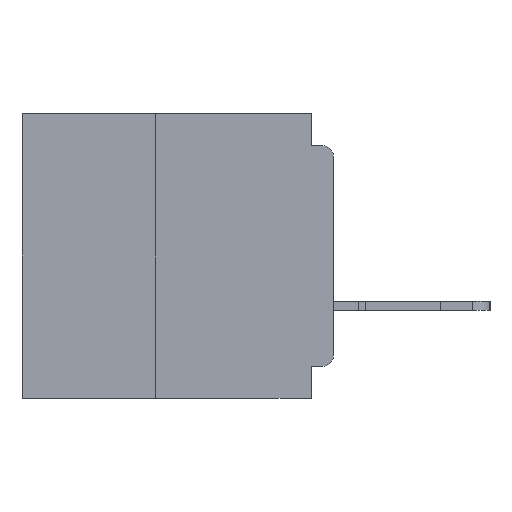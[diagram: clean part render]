
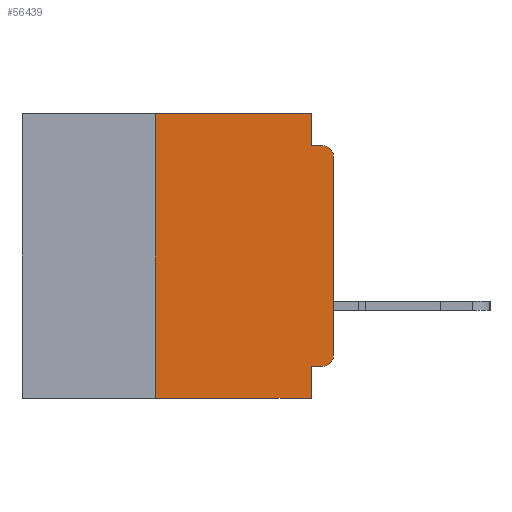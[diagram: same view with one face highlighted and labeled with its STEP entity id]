
A CAD part, left-side view. The second image highlights one B-rep face of the part: STEP entity #56439.
In plain terms, the highlighted planar face has unit normal (-1, 0, 0).
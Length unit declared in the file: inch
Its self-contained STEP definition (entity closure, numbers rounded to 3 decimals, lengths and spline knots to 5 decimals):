
#429 = CARTESIAN_POINT ( 'NONE',  ( 0., 0.015, -0.34 ) ) ;
#553 = EDGE_CURVE ( 'NONE', #53298, #14207, #32609, .T. ) ;
#2120 = PLANE ( 'NONE',  #48330 ) ;
#2488 = VERTEX_POINT ( 'NONE', #15504 ) ;
#4151 = FACE_OUTER_BOUND ( 'NONE', #9456, .T. ) ;
#4374 = ORIENTED_EDGE ( 'NONE', *, *, #48989, .F. ) ;
#4821 = CARTESIAN_POINT ( 'NONE',  ( 0., 0., -0.355 ) ) ;
#5250 = DIRECTION ( 'NONE',  ( 0., 0., -1. ) ) ;
#6593 = CARTESIAN_POINT ( 'NONE',  ( 0., 0., -0.34 ) ) ;
#6681 = VECTOR ( 'NONE', #27351, 39.37008 ) ;
#7150 = EDGE_CURVE ( 'NONE', #27262, #56945, #47640, .T. ) ;
#8183 = DIRECTION ( 'NONE',  ( -1., 0., 0. ) ) ;
#8783 = LINE ( 'NONE', #46534, #43451 ) ;
#9456 = EDGE_LOOP ( 'NONE', ( #33211, #60816, #21911, #58222, #13278, #57646, #57521, #50577, #4374, #11976 ) ) ;
#11715 = DIRECTION ( 'NONE',  ( 0., 0., -1. ) ) ;
#11976 = ORIENTED_EDGE ( 'NONE', *, *, #42810, .T. ) ;
#13278 = ORIENTED_EDGE ( 'NONE', *, *, #52804, .F. ) ;
#13912 = CARTESIAN_POINT ( 'NONE',  ( 0., 0.015, -0.045 ) ) ;
#14038 = VERTEX_POINT ( 'NONE', #56969 ) ;
#14207 = VERTEX_POINT ( 'NONE', #29874 ) ;
#15504 = CARTESIAN_POINT ( 'NONE',  ( 0., 0.031, -0.045 ) ) ;
#15814 = LINE ( 'NONE', #4821, #56228 ) ;
#18569 = VECTOR ( 'NONE', #18766, 39.37008 ) ;
#18766 = DIRECTION ( 'NONE',  ( 0., 0., 1. ) ) ;
#20874 = VECTOR ( 'NONE', #21956, 39.37008 ) ;
#21039 = DIRECTION ( 'NONE',  ( 0., -1., 0. ) ) ;
#21911 = ORIENTED_EDGE ( 'NONE', *, *, #32729, .F. ) ;
#21956 = DIRECTION ( 'NONE',  ( 0., -1., 0. ) ) ;
#22276 = CARTESIAN_POINT ( 'NONE',  ( 0., 0.25, -0.4 ) ) ;
#22679 = CIRCLE ( 'NONE', #32626, 0.015 ) ;
#27262 = VERTEX_POINT ( 'NONE', #22276 ) ;
#27351 = DIRECTION ( 'NONE',  ( 0., 0., 1. ) ) ;
#27953 = EDGE_CURVE ( 'NONE', #27262, #37650, #56746, .T. ) ;
#29874 = CARTESIAN_POINT ( 'NONE',  ( 0., 0., -0.06 ) ) ;
#30719 = CARTESIAN_POINT ( 'NONE',  ( 0., 0.031, -0.355 ) ) ;
#31317 = VECTOR ( 'NONE', #59017, 39.37008 ) ;
#31928 = CIRCLE ( 'NONE', #54908, 0.015 ) ;
#32609 = LINE ( 'NONE', #42254, #18569 ) ;
#32626 = AXIS2_PLACEMENT_3D ( 'NONE', #36455, #8183, #41176 ) ;
#32729 = EDGE_CURVE ( 'NONE', #2488, #40992, #33413, .T. ) ;
#33211 = ORIENTED_EDGE ( 'NONE', *, *, #553, .T. ) ;
#33413 = LINE ( 'NONE', #40703, #20874 ) ;
#33544 = DIRECTION ( 'NONE',  ( -1., 0., 0. ) ) ;
#35207 = CARTESIAN_POINT ( 'NONE',  ( 0., 0.437, 0. ) ) ;
#35329 = DIRECTION ( 'NONE',  ( 0., -1., 0. ) ) ;
#36455 = CARTESIAN_POINT ( 'NONE',  ( 0., 0.015, -0.06 ) ) ;
#36514 = VERTEX_POINT ( 'NONE', #30719 ) ;
#36623 = EDGE_CURVE ( 'NONE', #14207, #40992, #22679, .T. ) ;
#37320 = DIRECTION ( 'NONE',  ( 0., 0., -1. ) ) ;
#37650 = VERTEX_POINT ( 'NONE', #46918 ) ;
#37883 = DIRECTION ( 'NONE',  ( 0., 1., 0. ) ) ;
#39793 = CARTESIAN_POINT ( 'NONE',  ( 0., 0.437, -0.4 ) ) ;
#39947 = DIRECTION ( 'NONE',  ( 1., 0., 0. ) ) ;
#40005 = CARTESIAN_POINT ( 'NONE',  ( 0., 0.031, -0.4 ) ) ;
#40703 = CARTESIAN_POINT ( 'NONE',  ( 0., 0., -0.045 ) ) ;
#40992 = VERTEX_POINT ( 'NONE', #13912 ) ;
#41176 = DIRECTION ( 'NONE',  ( 0., 0., -1. ) ) ;
#42254 = CARTESIAN_POINT ( 'NONE',  ( 0., 0., 0. ) ) ;
#42810 = EDGE_CURVE ( 'NONE', #55442, #53298, #31928, .T. ) ;
#43451 = VECTOR ( 'NONE', #37320, 39.37008 ) ;
#43808 = LINE ( 'NONE', #40005, #31317 ) ;
#44564 = CARTESIAN_POINT ( 'NONE',  ( 0., 0.437, 0. ) ) ;
#46022 = CARTESIAN_POINT ( 'NONE',  ( 0., 0.25, -0.4 ) ) ;
#46534 = CARTESIAN_POINT ( 'NONE',  ( 0., 0.031, 0. ) ) ;
#46918 = CARTESIAN_POINT ( 'NONE',  ( 0., 0.25, 0. ) ) ;
#47640 = LINE ( 'NONE', #39793, #55677 ) ;
#48330 = AXIS2_PLACEMENT_3D ( 'NONE', #35207, #39947, #11715 ) ;
#48989 = EDGE_CURVE ( 'NONE', #55442, #36514, #15814, .T. ) ;
#50292 = CARTESIAN_POINT ( 'NONE',  ( 0., 0.015, -0.355 ) ) ;
#50577 = ORIENTED_EDGE ( 'NONE', *, *, #54080, .F. ) ;
#52804 = EDGE_CURVE ( 'NONE', #37650, #14038, #60818, .T. ) ;
#53298 = VERTEX_POINT ( 'NONE', #6593 ) ;
#54080 = EDGE_CURVE ( 'NONE', #36514, #56945, #43808, .T. ) ;
#54908 = AXIS2_PLACEMENT_3D ( 'NONE', #429, #33544, #5250 ) ;
#55442 = VERTEX_POINT ( 'NONE', #50292 ) ;
#55677 = VECTOR ( 'NONE', #21039, 39.37008 ) ;
#55811 = CARTESIAN_POINT ( 'NONE',  ( 0., 0.031, -0.4 ) ) ;
#56228 = VECTOR ( 'NONE', #37883, 39.37008 ) ;
#56439 = ADVANCED_FACE ( 'NONE', ( #4151 ), #2120, .F. ) ;
#56746 = LINE ( 'NONE', #46022, #6681 ) ;
#56945 = VERTEX_POINT ( 'NONE', #55811 ) ;
#56969 = CARTESIAN_POINT ( 'NONE',  ( 0., 0.031, 0. ) ) ;
#57521 = ORIENTED_EDGE ( 'NONE', *, *, #7150, .T. ) ;
#57646 = ORIENTED_EDGE ( 'NONE', *, *, #27953, .F. ) ;
#58222 = ORIENTED_EDGE ( 'NONE', *, *, #60016, .F. ) ;
#59017 = DIRECTION ( 'NONE',  ( 0., 0., -1. ) ) ;
#59346 = VECTOR ( 'NONE', #35329, 39.37008 ) ;
#60016 = EDGE_CURVE ( 'NONE', #14038, #2488, #8783, .T. ) ;
#60816 = ORIENTED_EDGE ( 'NONE', *, *, #36623, .T. ) ;
#60818 = LINE ( 'NONE', #44564, #59346 ) ;
